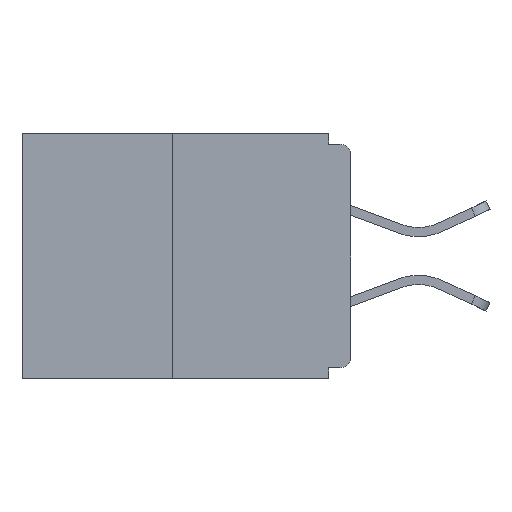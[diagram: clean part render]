
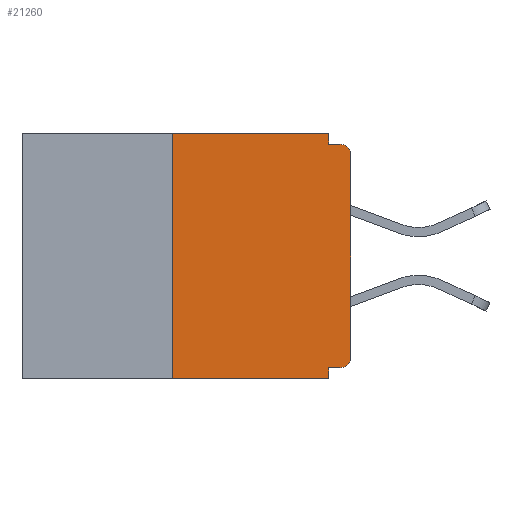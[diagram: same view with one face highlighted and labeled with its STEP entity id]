
A CAD part, left-side view. The second image highlights one B-rep face of the part: STEP entity #21260.
In plain terms, the highlighted planar face has unit normal (-1, 0, 0).
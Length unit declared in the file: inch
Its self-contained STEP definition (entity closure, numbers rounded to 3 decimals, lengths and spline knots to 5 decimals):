
#181 = ORIENTED_EDGE ( 'NONE', *, *, #19818, .T. ) ;
#366 = LINE ( 'NONE', #8191, #10434 ) ;
#468 = ORIENTED_EDGE ( 'NONE', *, *, #6536, .T. ) ;
#687 = ORIENTED_EDGE ( 'NONE', *, *, #5453, .F. ) ;
#939 = DIRECTION ( 'NONE',  ( 0., 0., -1. ) ) ;
#1995 = ORIENTED_EDGE ( 'NONE', *, *, #7515, .F. ) ;
#2365 = EDGE_LOOP ( 'NONE', ( #17556, #687, #468, #14361, #1995, #18531, #181, #22640, #20174, #5406 ) ) ;
#2475 = DIRECTION ( 'NONE',  ( -1., 0., 0. ) ) ;
#2508 = CARTESIAN_POINT ( 'NONE',  ( 0., 0.031, -0.328 ) ) ;
#2664 = DIRECTION ( 'NONE',  ( -1., 0., 0. ) ) ;
#2849 = LINE ( 'NONE', #13209, #12606 ) ;
#2851 = CARTESIAN_POINT ( 'NONE',  ( 0., 0., -0.03 ) ) ;
#2874 = DIRECTION ( 'NONE',  ( 0., 0., -1. ) ) ;
#2989 = VERTEX_POINT ( 'NONE', #9756 ) ;
#3778 = VERTEX_POINT ( 'NONE', #2508 ) ;
#3806 = VERTEX_POINT ( 'NONE', #8764 ) ;
#4282 = VECTOR ( 'NONE', #26476, 39.37008 ) ;
#4584 = VECTOR ( 'NONE', #14016, 39.37008 ) ;
#5056 = PLANE ( 'NONE',  #25055 ) ;
#5191 = CARTESIAN_POINT ( 'NONE',  ( 0., 0.25, -0.343 ) ) ;
#5406 = ORIENTED_EDGE ( 'NONE', *, *, #23461, .F. ) ;
#5453 = EDGE_CURVE ( 'NONE', #15239, #3806, #25003, .T. ) ;
#5630 = VERTEX_POINT ( 'NONE', #9034 ) ;
#5921 = LINE ( 'NONE', #24464, #4282 ) ;
#5997 = DIRECTION ( 'NONE',  ( 0., 1., 0. ) ) ;
#6225 = AXIS2_PLACEMENT_3D ( 'NONE', #9094, #2664, #939 ) ;
#6536 = EDGE_CURVE ( 'NONE', #15239, #17122, #15266, .T. ) ;
#6561 = DIRECTION ( 'NONE',  ( 0., 0., -1. ) ) ;
#6836 = VECTOR ( 'NONE', #19626, 39.37008 ) ;
#6945 = CARTESIAN_POINT ( 'NONE',  ( 0., 0.46, 0. ) ) ;
#7069 = CARTESIAN_POINT ( 'NONE',  ( 0., 0.015, -0.328 ) ) ;
#7244 = CARTESIAN_POINT ( 'NONE',  ( 0., 0.031, -0.015 ) ) ;
#7515 = EDGE_CURVE ( 'NONE', #24040, #3778, #366, .T. ) ;
#8191 = CARTESIAN_POINT ( 'NONE',  ( 0., 0., -0.328 ) ) ;
#8417 = VECTOR ( 'NONE', #13429, 39.37008 ) ;
#8764 = CARTESIAN_POINT ( 'NONE',  ( 0., 0.25, 0. ) ) ;
#9034 = CARTESIAN_POINT ( 'NONE',  ( 0., 0., -0.313 ) ) ;
#9092 = DIRECTION ( 'NONE',  ( 0., -1., 0. ) ) ;
#9094 = CARTESIAN_POINT ( 'NONE',  ( 0., 0.015, -0.313 ) ) ;
#9224 = DIRECTION ( 'NONE',  ( 1., 0., 0. ) ) ;
#9384 = EDGE_CURVE ( 'NONE', #3806, #2989, #2849, .T. ) ;
#9756 = CARTESIAN_POINT ( 'NONE',  ( 0., 0.031, 0. ) ) ;
#10393 = EDGE_CURVE ( 'NONE', #3778, #17122, #13843, .T. ) ;
#10434 = VECTOR ( 'NONE', #5997, 39.37008 ) ;
#11874 = VERTEX_POINT ( 'NONE', #2851 ) ;
#12606 = VECTOR ( 'NONE', #9092, 39.37008 ) ;
#13209 = CARTESIAN_POINT ( 'NONE',  ( 0., 0.46, 0. ) ) ;
#13334 = CARTESIAN_POINT ( 'NONE',  ( 0., 0., -0.015 ) ) ;
#13429 = DIRECTION ( 'NONE',  ( 0., -1., 0. ) ) ;
#13704 = LINE ( 'NONE', #13334, #6836 ) ;
#13830 = EDGE_CURVE ( 'NONE', #17212, #20507, #13704, .T. ) ;
#13843 = LINE ( 'NONE', #22575, #26822 ) ;
#14016 = DIRECTION ( 'NONE',  ( 0., 0., 1. ) ) ;
#14194 = DIRECTION ( 'NONE',  ( 0., 0., -1. ) ) ;
#14293 = CARTESIAN_POINT ( 'NONE',  ( 0., 0.015, -0.015 ) ) ;
#14361 = ORIENTED_EDGE ( 'NONE', *, *, #10393, .F. ) ;
#14512 = FACE_OUTER_BOUND ( 'NONE', #2365, .T. ) ;
#15239 = VERTEX_POINT ( 'NONE', #5191 ) ;
#15266 = LINE ( 'NONE', #25999, #8417 ) ;
#15460 = AXIS2_PLACEMENT_3D ( 'NONE', #17112, #2475, #6561 ) ;
#16054 = VECTOR ( 'NONE', #17513, 39.37008 ) ;
#16292 = CARTESIAN_POINT ( 'NONE',  ( 0., 0.25, 0. ) ) ;
#17112 = CARTESIAN_POINT ( 'NONE',  ( 0., 0.015, -0.03 ) ) ;
#17122 = VERTEX_POINT ( 'NONE', #23742 ) ;
#17212 = VERTEX_POINT ( 'NONE', #7244 ) ;
#17513 = DIRECTION ( 'NONE',  ( 0., 0., 1. ) ) ;
#17556 = ORIENTED_EDGE ( 'NONE', *, *, #9384, .F. ) ;
#17561 = EDGE_CURVE ( 'NONE', #24040, #5630, #26465, .T. ) ;
#18531 = ORIENTED_EDGE ( 'NONE', *, *, #17561, .T. ) ;
#19626 = DIRECTION ( 'NONE',  ( 0., -1., 0. ) ) ;
#19818 = EDGE_CURVE ( 'NONE', #5630, #11874, #26100, .T. ) ;
#20051 = CIRCLE ( 'NONE', #15460, 0.015 ) ;
#20174 = ORIENTED_EDGE ( 'NONE', *, *, #13830, .F. ) ;
#20507 = VERTEX_POINT ( 'NONE', #14293 ) ;
#21260 = ADVANCED_FACE ( 'NONE', ( #14512 ), #5056, .F. ) ;
#22575 = CARTESIAN_POINT ( 'NONE',  ( 0., 0.031, -0.343 ) ) ;
#22640 = ORIENTED_EDGE ( 'NONE', *, *, #25382, .T. ) ;
#23461 = EDGE_CURVE ( 'NONE', #2989, #17212, #5921, .T. ) ;
#23742 = CARTESIAN_POINT ( 'NONE',  ( 0., 0.031, -0.343 ) ) ;
#23797 = CARTESIAN_POINT ( 'NONE',  ( 0., 0., 0. ) ) ;
#24040 = VERTEX_POINT ( 'NONE', #7069 ) ;
#24464 = CARTESIAN_POINT ( 'NONE',  ( 0., 0.031, 0. ) ) ;
#25003 = LINE ( 'NONE', #16292, #4584 ) ;
#25055 = AXIS2_PLACEMENT_3D ( 'NONE', #6945, #9224, #2874 ) ;
#25382 = EDGE_CURVE ( 'NONE', #11874, #20507, #20051, .T. ) ;
#25999 = CARTESIAN_POINT ( 'NONE',  ( 0., 0.46, -0.343 ) ) ;
#26100 = LINE ( 'NONE', #23797, #16054 ) ;
#26465 = CIRCLE ( 'NONE', #6225, 0.015 ) ;
#26476 = DIRECTION ( 'NONE',  ( 0., 0., -1. ) ) ;
#26822 = VECTOR ( 'NONE', #14194, 39.37008 ) ;
